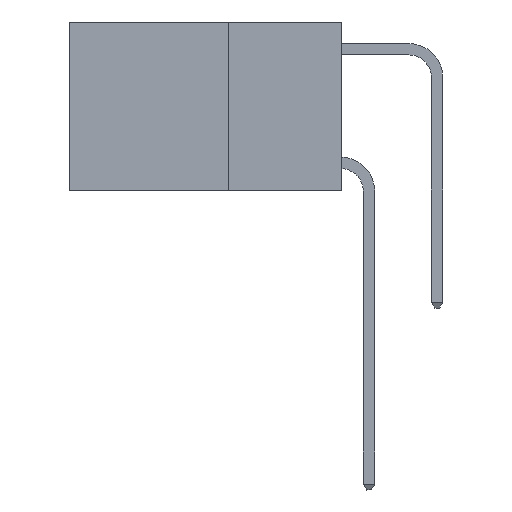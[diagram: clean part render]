
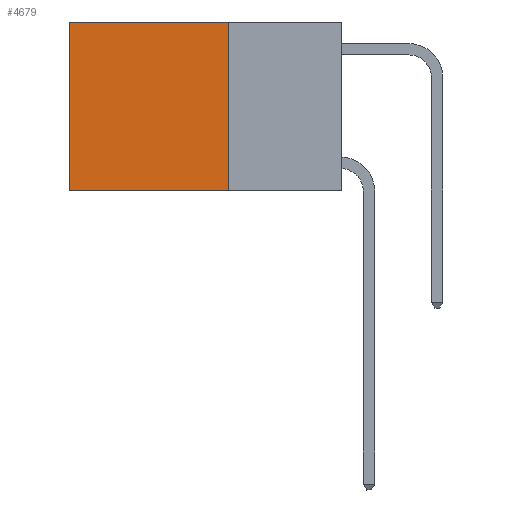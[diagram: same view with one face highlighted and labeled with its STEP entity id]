
A CAD part, left-side view. The second image highlights one B-rep face of the part: STEP entity #4679.
In plain terms, the highlighted planar face has unit normal (-1, 0, 0).
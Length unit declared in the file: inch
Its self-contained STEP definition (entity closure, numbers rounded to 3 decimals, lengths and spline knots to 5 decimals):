
#121 = FACE_OUTER_BOUND ( 'NONE', #5345, .T. ) ;
#741 = EDGE_CURVE ( 'NONE', #6727, #11832, #15187, .T. ) ;
#1184 = VERTEX_POINT ( 'NONE', #13166 ) ;
#2762 = VECTOR ( 'NONE', #12812, 39.37008 ) ;
#3565 = DIRECTION ( 'NONE',  ( 0., 0., -1. ) ) ;
#4007 = CARTESIAN_POINT ( 'NONE',  ( 0.2625, 0.25, 0. ) ) ;
#4026 = VECTOR ( 'NONE', #15164, 39.37008 ) ;
#4679 = ADVANCED_FACE ( 'NONE', ( #121 ), #13522, .F. ) ;
#5345 = EDGE_LOOP ( 'NONE', ( #10006, #15013, #16769, #14244 ) ) ;
#6727 = VERTEX_POINT ( 'NONE', #18839 ) ;
#6849 = VERTEX_POINT ( 'NONE', #23465 ) ;
#7252 = VECTOR ( 'NONE', #22002, 39.37008 ) ;
#7526 = CARTESIAN_POINT ( 'NONE',  ( 0.2625, 0.25, 0. ) ) ;
#7759 = EDGE_CURVE ( 'NONE', #6849, #6727, #23164, .T. ) ;
#8743 = LINE ( 'NONE', #22256, #7252 ) ;
#9511 = EDGE_CURVE ( 'NONE', #6849, #1184, #8743, .T. ) ;
#10006 = ORIENTED_EDGE ( 'NONE', *, *, #741, .T. ) ;
#10241 = DIRECTION ( 'NONE',  ( 1., 0., 0. ) ) ;
#11832 = VERTEX_POINT ( 'NONE', #20803 ) ;
#12258 = DIRECTION ( 'NONE',  ( 0., 0., -1. ) ) ;
#12812 = DIRECTION ( 'NONE',  ( 0., 1., 0. ) ) ;
#13166 = CARTESIAN_POINT ( 'NONE',  ( 0.2625, 0.25, -0.37 ) ) ;
#13522 = PLANE ( 'NONE',  #14853 ) ;
#14244 = ORIENTED_EDGE ( 'NONE', *, *, #7759, .T. ) ;
#14853 = AXIS2_PLACEMENT_3D ( 'NONE', #4007, #10241, #12258 ) ;
#15013 = ORIENTED_EDGE ( 'NONE', *, *, #20921, .F. ) ;
#15164 = DIRECTION ( 'NONE',  ( 0., 1., 0. ) ) ;
#15187 = LINE ( 'NONE', #20937, #16268 ) ;
#16268 = VECTOR ( 'NONE', #3565, 39.37008 ) ;
#16338 = LINE ( 'NONE', #16443, #2762 ) ;
#16443 = CARTESIAN_POINT ( 'NONE',  ( 0.2625, 0.25, -0.37 ) ) ;
#16769 = ORIENTED_EDGE ( 'NONE', *, *, #9511, .F. ) ;
#18839 = CARTESIAN_POINT ( 'NONE',  ( 0.2625, 0.6, 0. ) ) ;
#20803 = CARTESIAN_POINT ( 'NONE',  ( 0.2625, 0.6, -0.37 ) ) ;
#20921 = EDGE_CURVE ( 'NONE', #1184, #11832, #16338, .T. ) ;
#20937 = CARTESIAN_POINT ( 'NONE',  ( 0.2625, 0.6, 0. ) ) ;
#22002 = DIRECTION ( 'NONE',  ( 0., 0., -1. ) ) ;
#22256 = CARTESIAN_POINT ( 'NONE',  ( 0.2625, 0.25, 0. ) ) ;
#23164 = LINE ( 'NONE', #7526, #4026 ) ;
#23465 = CARTESIAN_POINT ( 'NONE',  ( 0.2625, 0.25, 0. ) ) ;
